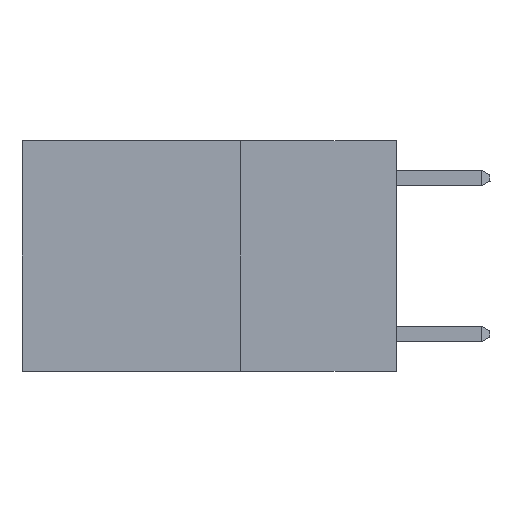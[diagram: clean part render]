
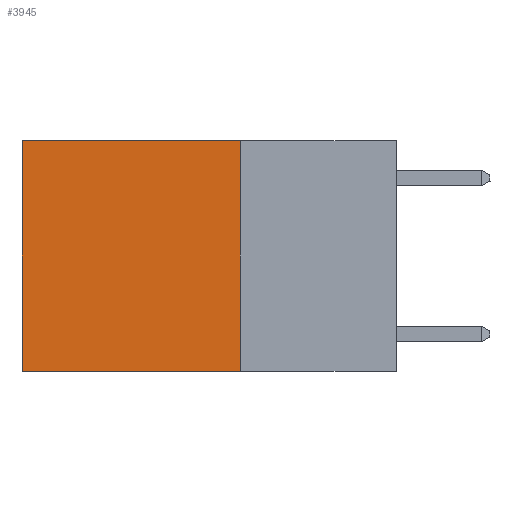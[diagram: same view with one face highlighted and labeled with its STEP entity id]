
A CAD part, left-side view. The second image highlights one B-rep face of the part: STEP entity #3945.
In plain terms, the highlighted planar face has unit normal (-1, 0, 0).
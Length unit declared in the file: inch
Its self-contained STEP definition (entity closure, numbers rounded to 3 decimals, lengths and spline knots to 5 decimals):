
#336 = CARTESIAN_POINT ( 'NONE',  ( 0.2625, 0.6, -0.37 ) ) ;
#588 = EDGE_CURVE ( 'NONE', #4892, #8347, #1003, .T. ) ;
#960 = EDGE_CURVE ( 'NONE', #1014, #8347, #9543, .T. ) ;
#1003 = LINE ( 'NONE', #10163, #12204 ) ;
#1014 = VERTEX_POINT ( 'NONE', #7799 ) ;
#1529 = CARTESIAN_POINT ( 'NONE',  ( 0.2625, 0.25, -0.37 ) ) ;
#1966 = DIRECTION ( 'NONE',  ( 1., 0., 0. ) ) ;
#2808 = DIRECTION ( 'NONE',  ( 0., 0., -1. ) ) ;
#3147 = VECTOR ( 'NONE', #4683, 39.37008 ) ;
#3218 = CARTESIAN_POINT ( 'NONE',  ( 0.2625, 0.25, 0. ) ) ;
#3699 = CARTESIAN_POINT ( 'NONE',  ( 0.2625, 0.6, 0. ) ) ;
#3945 = ADVANCED_FACE ( 'NONE', ( #5037 ), #6194, .F. ) ;
#4026 = EDGE_CURVE ( 'NONE', #10689, #4892, #13301, .T. ) ;
#4046 = CARTESIAN_POINT ( 'NONE',  ( 0.2625, 0.25, 0. ) ) ;
#4683 = DIRECTION ( 'NONE',  ( 0., 1., 0. ) ) ;
#4892 = VERTEX_POINT ( 'NONE', #3699 ) ;
#5037 = FACE_OUTER_BOUND ( 'NONE', #7463, .T. ) ;
#6194 = PLANE ( 'NONE',  #10732 ) ;
#7100 = VECTOR ( 'NONE', #7170, 39.37008 ) ;
#7170 = DIRECTION ( 'NONE',  ( 0., 1., 0. ) ) ;
#7463 = EDGE_LOOP ( 'NONE', ( #11471, #7512, #10664, #12535 ) ) ;
#7512 = ORIENTED_EDGE ( 'NONE', *, *, #960, .F. ) ;
#7799 = CARTESIAN_POINT ( 'NONE',  ( 0.2625, 0.25, -0.37 ) ) ;
#8347 = VERTEX_POINT ( 'NONE', #336 ) ;
#9543 = LINE ( 'NONE', #1529, #3147 ) ;
#10163 = CARTESIAN_POINT ( 'NONE',  ( 0.2625, 0.6, 0. ) ) ;
#10242 = CARTESIAN_POINT ( 'NONE',  ( 0.2625, 0.25, 0. ) ) ;
#10598 = EDGE_CURVE ( 'NONE', #10689, #1014, #12060, .T. ) ;
#10664 = ORIENTED_EDGE ( 'NONE', *, *, #10598, .F. ) ;
#10689 = VERTEX_POINT ( 'NONE', #3218 ) ;
#10732 = AXIS2_PLACEMENT_3D ( 'NONE', #10242, #1966, #11134 ) ;
#11134 = DIRECTION ( 'NONE',  ( 0., 0., -1. ) ) ;
#11192 = VECTOR ( 'NONE', #2808, 39.37008 ) ;
#11325 = DIRECTION ( 'NONE',  ( 0., 0., -1. ) ) ;
#11471 = ORIENTED_EDGE ( 'NONE', *, *, #588, .T. ) ;
#11881 = CARTESIAN_POINT ( 'NONE',  ( 0.2625, 0.25, 0. ) ) ;
#12060 = LINE ( 'NONE', #11881, #11192 ) ;
#12204 = VECTOR ( 'NONE', #11325, 39.37008 ) ;
#12535 = ORIENTED_EDGE ( 'NONE', *, *, #4026, .T. ) ;
#13301 = LINE ( 'NONE', #4046, #7100 ) ;
